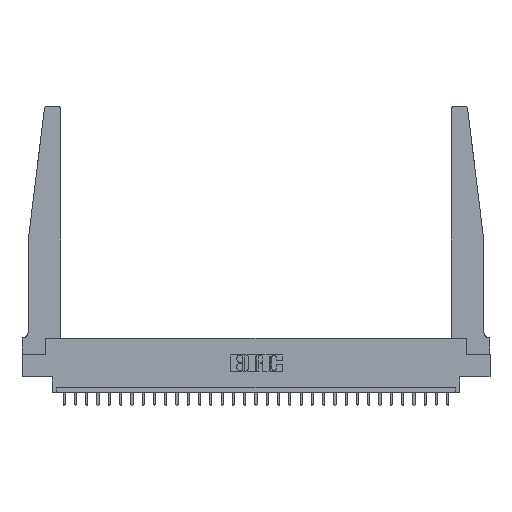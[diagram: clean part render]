
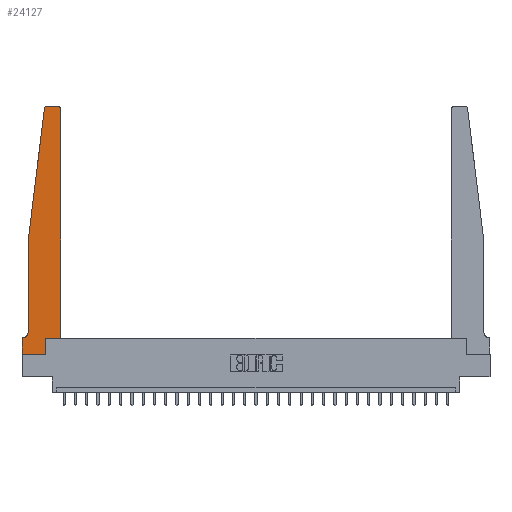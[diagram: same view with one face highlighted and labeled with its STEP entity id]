
A CAD part, top view. The second image highlights one B-rep face of the part: STEP entity #24127.
In plain terms, the highlighted planar face has unit normal (0, 0, 1).
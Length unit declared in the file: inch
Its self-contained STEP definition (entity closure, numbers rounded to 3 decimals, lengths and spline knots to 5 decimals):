
#28 = CARTESIAN_POINT ( 'NONE',  ( 0.425, 2.72, 0.37 ) ) ;
#62 = DIRECTION ( 'NONE',  ( 1., 0., 0. ) ) ;
#369 = CARTESIAN_POINT ( 'NONE',  ( 0.27653, 2.72, 0.37 ) ) ;
#948 = VERTEX_POINT ( 'NONE', #4933 ) ;
#1172 = DIRECTION ( 'NONE',  ( -1., 0., 0. ) ) ;
#1493 = DIRECTION ( 'NONE',  ( -1., 0., 0. ) ) ;
#1521 = DIRECTION ( 'NONE',  ( 0., -1., 0. ) ) ;
#1719 = VECTOR ( 'NONE', #1172, 39.37008 ) ;
#1916 = CARTESIAN_POINT ( 'NONE',  ( 0.2605, 0., 0.37 ) ) ;
#1990 = EDGE_CURVE ( 'NONE', #948, #16462, #12123, .T. ) ;
#2088 = CARTESIAN_POINT ( 'NONE',  ( 0., 0., 0.37 ) ) ;
#2230 = EDGE_CURVE ( 'NONE', #6884, #18299, #11782, .T. ) ;
#2303 = LINE ( 'NONE', #14373, #18293 ) ;
#2673 = LINE ( 'NONE', #7845, #20309 ) ;
#3024 = VECTOR ( 'NONE', #20373, 39.37008 ) ;
#3148 = CARTESIAN_POINT ( 'NONE',  ( 0.015, 0.2375, 0.37 ) ) ;
#3224 = DIRECTION ( 'NONE',  ( 0., 0., 1. ) ) ;
#3225 = EDGE_CURVE ( 'NONE', #10870, #948, #8050, .T. ) ;
#3558 = ORIENTED_EDGE ( 'NONE', *, *, #17348, .T. ) ;
#4013 = CARTESIAN_POINT ( 'NONE',  ( 0.395, 2.75, 0.37 ) ) ;
#4845 = EDGE_CURVE ( 'NONE', #10938, #21940, #6648, .T. ) ;
#4933 = CARTESIAN_POINT ( 'NONE',  ( 0., 0., 0.37 ) ) ;
#4984 = VERTEX_POINT ( 'NONE', #8593 ) ;
#5244 = VERTEX_POINT ( 'NONE', #26669 ) ;
#5290 = CARTESIAN_POINT ( 'NONE',  ( 0.425, 0.18, 0.37 ) ) ;
#5381 = EDGE_CURVE ( 'NONE', #18299, #21792, #2303, .T. ) ;
#5543 = PLANE ( 'NONE',  #23813 ) ;
#5821 = DIRECTION ( 'NONE',  ( -1., 0., 0. ) ) ;
#6491 = CIRCLE ( 'NONE', #14230, 0.03 ) ;
#6648 = LINE ( 'NONE', #12032, #11327 ) ;
#6884 = VERTEX_POINT ( 'NONE', #28 ) ;
#7191 = CARTESIAN_POINT ( 'NONE',  ( 0.395, 2.72, 0.37 ) ) ;
#7415 = CARTESIAN_POINT ( 'NONE',  ( 0., 0.1875, 0.37 ) ) ;
#7503 = DIRECTION ( 'NONE',  ( 0., 0., -1. ) ) ;
#7845 = CARTESIAN_POINT ( 'NONE',  ( 0.065, 1.25, 0.37 ) ) ;
#8050 = LINE ( 'NONE', #25909, #23415 ) ;
#8593 = CARTESIAN_POINT ( 'NONE',  ( 0.015, 0.1875, 0.37 ) ) ;
#9238 = DIRECTION ( 'NONE',  ( 0., 0., 1. ) ) ;
#9253 = CARTESIAN_POINT ( 'NONE',  ( 0.24675, 2.72367, 0.37 ) ) ;
#9532 = ORIENTED_EDGE ( 'NONE', *, *, #1990, .T. ) ;
#10089 = LINE ( 'NONE', #18092, #1719 ) ;
#10191 = DIRECTION ( 'NONE',  ( -0.122, -0.992, 0. ) ) ;
#10409 = ORIENTED_EDGE ( 'NONE', *, *, #4845, .T. ) ;
#10505 = ORIENTED_EDGE ( 'NONE', *, *, #3225, .T. ) ;
#10870 = VERTEX_POINT ( 'NONE', #22350 ) ;
#10938 = VERTEX_POINT ( 'NONE', #26660 ) ;
#11327 = VECTOR ( 'NONE', #1521, 39.37008 ) ;
#11782 = CIRCLE ( 'NONE', #13826, 0.03 ) ;
#11956 = EDGE_CURVE ( 'NONE', #21940, #4984, #14426, .T. ) ;
#12032 = CARTESIAN_POINT ( 'NONE',  ( 0.065, 1.25, 0.37 ) ) ;
#12123 = LINE ( 'NONE', #2088, #24163 ) ;
#12501 = VERTEX_POINT ( 'NONE', #9253 ) ;
#13052 = DIRECTION ( 'NONE',  ( 0., -1., 0. ) ) ;
#13826 = AXIS2_PLACEMENT_3D ( 'NONE', #7191, #22196, #24361 ) ;
#13970 = DIRECTION ( 'NONE',  ( 1., 0., 0. ) ) ;
#14069 = EDGE_CURVE ( 'NONE', #23280, #6884, #27061, .T. ) ;
#14165 = DIRECTION ( 'NONE',  ( 0., 1., 0. ) ) ;
#14195 = EDGE_CURVE ( 'NONE', #16462, #5244, #15649, .T. ) ;
#14203 = ORIENTED_EDGE ( 'NONE', *, *, #11956, .T. ) ;
#14230 = AXIS2_PLACEMENT_3D ( 'NONE', #369, #9238, #15411 ) ;
#14373 = CARTESIAN_POINT ( 'NONE',  ( 0.25, 2.75, 0.37 ) ) ;
#14426 = CIRCLE ( 'NONE', #26396, 0.05 ) ;
#15411 = DIRECTION ( 'NONE',  ( 1., 0., 0. ) ) ;
#15649 = LINE ( 'NONE', #18840, #25733 ) ;
#15656 = ORIENTED_EDGE ( 'NONE', *, *, #14195, .T. ) ;
#15851 = CARTESIAN_POINT ( 'NONE',  ( 0.425, 0.18, 0.37 ) ) ;
#16462 = VERTEX_POINT ( 'NONE', #1916 ) ;
#17348 = EDGE_CURVE ( 'NONE', #12501, #10938, #2673, .T. ) ;
#18092 = CARTESIAN_POINT ( 'NONE',  ( 0.065, 0.1875, 0.37 ) ) ;
#18293 = VECTOR ( 'NONE', #1493, 39.37008 ) ;
#18299 = VERTEX_POINT ( 'NONE', #4013 ) ;
#18319 = ORIENTED_EDGE ( 'NONE', *, *, #2230, .T. ) ;
#18826 = DIRECTION ( 'NONE',  ( 1., 0., 0. ) ) ;
#18840 = CARTESIAN_POINT ( 'NONE',  ( 0.2605, 0.18, 0.37 ) ) ;
#19557 = CARTESIAN_POINT ( 'NONE',  ( 0.065, 0.2375, 0.37 ) ) ;
#19894 = ORIENTED_EDGE ( 'NONE', *, *, #23302, .T. ) ;
#20309 = VECTOR ( 'NONE', #10191, 39.37008 ) ;
#20315 = ORIENTED_EDGE ( 'NONE', *, *, #14069, .T. ) ;
#20373 = DIRECTION ( 'NONE',  ( 0., 1., 0. ) ) ;
#20758 = EDGE_CURVE ( 'NONE', #21792, #12501, #6491, .T. ) ;
#21792 = VERTEX_POINT ( 'NONE', #25502 ) ;
#21940 = VERTEX_POINT ( 'NONE', #19557 ) ;
#22196 = DIRECTION ( 'NONE',  ( 0., 0., 1. ) ) ;
#22350 = CARTESIAN_POINT ( 'NONE',  ( 0., 0.1875, 0.37 ) ) ;
#23265 = ORIENTED_EDGE ( 'NONE', *, *, #20758, .T. ) ;
#23280 = VERTEX_POINT ( 'NONE', #15851 ) ;
#23302 = EDGE_CURVE ( 'NONE', #4984, #10870, #10089, .T. ) ;
#23415 = VECTOR ( 'NONE', #13052, 39.37008 ) ;
#23813 = AXIS2_PLACEMENT_3D ( 'NONE', #7415, #3224, #13970 ) ;
#23815 = VECTOR ( 'NONE', #18826, 39.37008 ) ;
#24127 = ADVANCED_FACE ( 'NONE', ( #26189 ), #5543, .T. ) ;
#24163 = VECTOR ( 'NONE', #62, 39.37008 ) ;
#24361 = DIRECTION ( 'NONE',  ( 1., 0., 0. ) ) ;
#24512 = EDGE_CURVE ( 'NONE', #5244, #23280, #26832, .T. ) ;
#25502 = CARTESIAN_POINT ( 'NONE',  ( 0.27653, 2.75, 0.37 ) ) ;
#25698 = CARTESIAN_POINT ( 'NONE',  ( 0.425, 0.18, 0.37 ) ) ;
#25733 = VECTOR ( 'NONE', #14165, 39.37008 ) ;
#25909 = CARTESIAN_POINT ( 'NONE',  ( 0., 0., 0.37 ) ) ;
#26189 = FACE_OUTER_BOUND ( 'NONE', #27104, .T. ) ;
#26396 = AXIS2_PLACEMENT_3D ( 'NONE', #3148, #7503, #5821 ) ;
#26660 = CARTESIAN_POINT ( 'NONE',  ( 0.065, 1.25, 0.37 ) ) ;
#26669 = CARTESIAN_POINT ( 'NONE',  ( 0.2605, 0.18, 0.37 ) ) ;
#26832 = LINE ( 'NONE', #25698, #23815 ) ;
#26833 = ORIENTED_EDGE ( 'NONE', *, *, #5381, .T. ) ;
#27061 = LINE ( 'NONE', #5290, #3024 ) ;
#27104 = EDGE_LOOP ( 'NONE', ( #26833, #23265, #3558, #10409, #14203, #19894, #10505, #9532, #15656, #27302, #20315, #18319 ) ) ;
#27302 = ORIENTED_EDGE ( 'NONE', *, *, #24512, .T. ) ;
